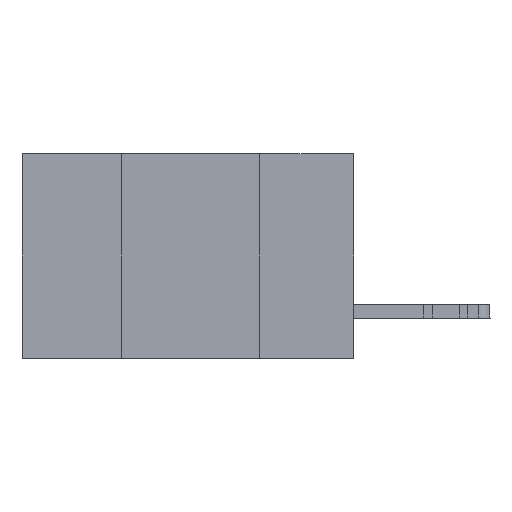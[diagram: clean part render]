
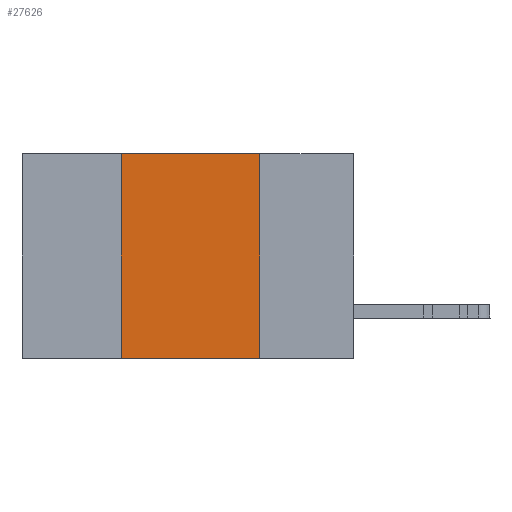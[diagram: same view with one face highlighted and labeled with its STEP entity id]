
A CAD part, left-side view. The second image highlights one B-rep face of the part: STEP entity #27626.
In plain terms, the highlighted planar face has unit normal (-1, 0, 0).
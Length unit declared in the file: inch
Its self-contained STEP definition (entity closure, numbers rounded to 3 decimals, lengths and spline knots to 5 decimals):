
#360 = VECTOR ( 'NONE', #29797, 39.37008 ) ;
#1180 = CARTESIAN_POINT ( 'NONE',  ( 0., 0.17, 0. ) ) ;
#1393 = VECTOR ( 'NONE', #4334, 39.37008 ) ;
#2927 = ORIENTED_EDGE ( 'NONE', *, *, #38403, .T. ) ;
#4111 = CARTESIAN_POINT ( 'NONE',  ( 0., 0.6, 0. ) ) ;
#4334 = DIRECTION ( 'NONE',  ( 0., -1., 0. ) ) ;
#5250 = LINE ( 'NONE', #25928, #43178 ) ;
#7712 = VERTEX_POINT ( 'NONE', #43538 ) ;
#9123 = ORIENTED_EDGE ( 'NONE', *, *, #25379, .F. ) ;
#11356 = VECTOR ( 'NONE', #34344, 39.37008 ) ;
#11413 = LINE ( 'NONE', #28096, #11356 ) ;
#11805 = LINE ( 'NONE', #22686, #360 ) ;
#12567 = EDGE_LOOP ( 'NONE', ( #13808, #9123, #43711, #2927 ) ) ;
#13808 = ORIENTED_EDGE ( 'NONE', *, *, #20607, .F. ) ;
#14282 = CARTESIAN_POINT ( 'NONE',  ( 0., 0.42, -0.37 ) ) ;
#14337 = CARTESIAN_POINT ( 'NONE',  ( 0., 0.17, -0.37 ) ) ;
#16469 = VERTEX_POINT ( 'NONE', #14282 ) ;
#20607 = EDGE_CURVE ( 'NONE', #20855, #28728, #5250, .T. ) ;
#20855 = VERTEX_POINT ( 'NONE', #1180 ) ;
#22588 = DIRECTION ( 'NONE',  ( 0., 0., -1. ) ) ;
#22686 = CARTESIAN_POINT ( 'NONE',  ( 0., 0.6, -0.37 ) ) ;
#25379 = EDGE_CURVE ( 'NONE', #7712, #20855, #31694, .T. ) ;
#25928 = CARTESIAN_POINT ( 'NONE',  ( 0., 0.17, 0. ) ) ;
#27072 = EDGE_CURVE ( 'NONE', #16469, #7712, #11413, .T. ) ;
#27626 = ADVANCED_FACE ( 'NONE', ( #33292 ), #41834, .F. ) ;
#28096 = CARTESIAN_POINT ( 'NONE',  ( 0., 0.42, 0. ) ) ;
#28728 = VERTEX_POINT ( 'NONE', #14337 ) ;
#29736 = CARTESIAN_POINT ( 'NONE',  ( 0., 0.6, 0. ) ) ;
#29797 = DIRECTION ( 'NONE',  ( 0., -1., 0. ) ) ;
#31694 = LINE ( 'NONE', #4111, #1393 ) ;
#33292 = FACE_OUTER_BOUND ( 'NONE', #12567, .T. ) ;
#34344 = DIRECTION ( 'NONE',  ( 0., 0., 1. ) ) ;
#35165 = DIRECTION ( 'NONE',  ( 1., 0., 0. ) ) ;
#36419 = DIRECTION ( 'NONE',  ( 0., 0., -1. ) ) ;
#38403 = EDGE_CURVE ( 'NONE', #16469, #28728, #11805, .T. ) ;
#41834 = PLANE ( 'NONE',  #43363 ) ;
#43178 = VECTOR ( 'NONE', #22588, 39.37008 ) ;
#43363 = AXIS2_PLACEMENT_3D ( 'NONE', #29736, #35165, #36419 ) ;
#43538 = CARTESIAN_POINT ( 'NONE',  ( 0., 0.42, 0. ) ) ;
#43711 = ORIENTED_EDGE ( 'NONE', *, *, #27072, .F. ) ;
